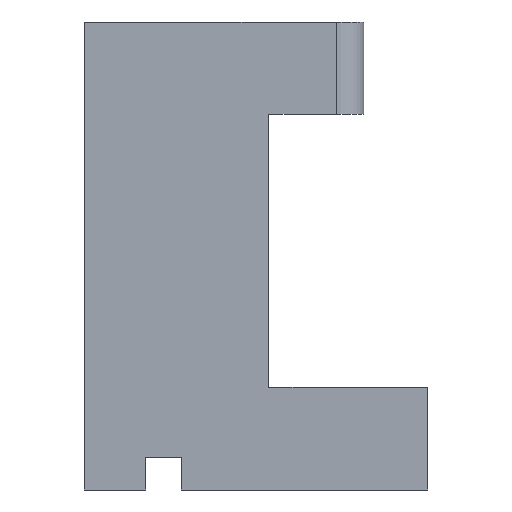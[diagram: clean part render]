
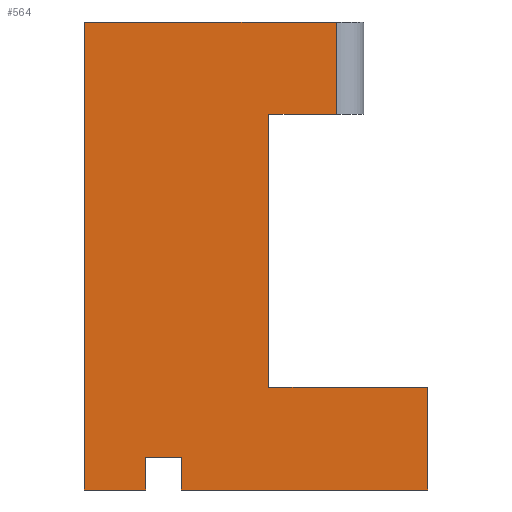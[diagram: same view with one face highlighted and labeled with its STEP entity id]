
A CAD part, front view. The second image highlights one B-rep face of the part: STEP entity #564.
In plain terms, the highlighted planar face has unit normal (0, -1, 0).
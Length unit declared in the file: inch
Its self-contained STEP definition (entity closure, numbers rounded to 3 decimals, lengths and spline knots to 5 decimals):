
#36=FACE_OUTER_BOUND('',#66,.T.);
#66=EDGE_LOOP('',(#399,#400,#401,#402,#403,#404,#405,#406,#407,#408,#409,
#410));
#125=LINE('',#836,#185);
#139=LINE('',#864,#199);
#140=LINE('',#866,#200);
#141=LINE('',#868,#201);
#142=LINE('',#870,#202);
#143=LINE('',#872,#203);
#144=LINE('',#874,#204);
#145=LINE('',#876,#205);
#146=LINE('',#878,#206);
#147=LINE('',#880,#207);
#148=LINE('',#882,#208);
#149=LINE('',#883,#209);
#185=VECTOR('',#669,0.3937);
#199=VECTOR('',#687,0.3937);
#200=VECTOR('',#688,0.3937);
#201=VECTOR('',#689,0.3937);
#202=VECTOR('',#690,0.3937);
#203=VECTOR('',#691,0.3937);
#204=VECTOR('',#692,0.3937);
#205=VECTOR('',#693,0.3937);
#206=VECTOR('',#694,0.3937);
#207=VECTOR('',#695,0.3937);
#208=VECTOR('',#696,0.3937);
#209=VECTOR('',#697,0.3937);
#246=VERTEX_POINT('',#832);
#248=VERTEX_POINT('',#835);
#260=VERTEX_POINT('',#863);
#261=VERTEX_POINT('',#865);
#262=VERTEX_POINT('',#867);
#263=VERTEX_POINT('',#869);
#264=VERTEX_POINT('',#871);
#265=VERTEX_POINT('',#873);
#266=VERTEX_POINT('',#875);
#267=VERTEX_POINT('',#877);
#268=VERTEX_POINT('',#879);
#269=VERTEX_POINT('',#881);
#302=EDGE_CURVE('',#248,#246,#125,.T.);
#316=EDGE_CURVE('',#260,#248,#139,.T.);
#317=EDGE_CURVE('',#261,#246,#140,.T.);
#318=EDGE_CURVE('',#261,#262,#141,.T.);
#319=EDGE_CURVE('',#262,#263,#142,.T.);
#320=EDGE_CURVE('',#263,#264,#143,.T.);
#321=EDGE_CURVE('',#265,#264,#144,.T.);
#322=EDGE_CURVE('',#265,#266,#145,.T.);
#323=EDGE_CURVE('',#266,#267,#146,.T.);
#324=EDGE_CURVE('',#267,#268,#147,.T.);
#325=EDGE_CURVE('',#269,#268,#148,.T.);
#326=EDGE_CURVE('',#260,#269,#149,.T.);
#399=ORIENTED_EDGE('',*,*,#316,.T.);
#400=ORIENTED_EDGE('',*,*,#302,.T.);
#401=ORIENTED_EDGE('',*,*,#317,.F.);
#402=ORIENTED_EDGE('',*,*,#318,.T.);
#403=ORIENTED_EDGE('',*,*,#319,.T.);
#404=ORIENTED_EDGE('',*,*,#320,.T.);
#405=ORIENTED_EDGE('',*,*,#321,.F.);
#406=ORIENTED_EDGE('',*,*,#322,.T.);
#407=ORIENTED_EDGE('',*,*,#323,.T.);
#408=ORIENTED_EDGE('',*,*,#324,.T.);
#409=ORIENTED_EDGE('',*,*,#325,.F.);
#410=ORIENTED_EDGE('',*,*,#326,.F.);
#545=PLANE('',#609);
#564=ADVANCED_FACE('',(#36),#545,.T.);
#609=AXIS2_PLACEMENT_3D('',#862,#685,#686);
#669=DIRECTION('',(0.,0.,1.));
#685=DIRECTION('center_axis',(0.,-1.,0.));
#686=DIRECTION('ref_axis',(0.,0.,-1.));
#687=DIRECTION('',(-1.,0.,0.));
#688=DIRECTION('',(-1.,0.,0.));
#689=DIRECTION('',(0.,0.,1.));
#690=DIRECTION('',(-1.,0.,0.));
#691=DIRECTION('',(0.,0.,-1.));
#692=DIRECTION('',(-1.,0.,0.));
#693=DIRECTION('',(0.,0.,1.));
#694=DIRECTION('',(1.,0.,0.));
#695=DIRECTION('',(0.,0.,-1.));
#696=DIRECTION('',(-1.,0.,0.));
#697=DIRECTION('',(0.,0.,-1.));
#832=CARTESIAN_POINT('',(-9.86369,-2.02165,3.12));
#835=CARTESIAN_POINT('',(-9.86369,-2.02165,1.27));
#836=CARTESIAN_POINT('',(-9.86369,-2.02165,1.70441));
#862=CARTESIAN_POINT('Origin',(-10.08567,-2.02165,2.08381));
#863=CARTESIAN_POINT('',(-8.78869,-2.02165,1.27));
#864=CARTESIAN_POINT('',(-9.93718,-2.02165,1.27));
#865=CARTESIAN_POINT('',(-9.40669,-2.02165,3.12));
#866=CARTESIAN_POINT('',(-9.15669,-2.02165,3.12));
#867=CARTESIAN_POINT('',(-9.40669,-2.02165,3.745));
#868=CARTESIAN_POINT('',(-9.40669,-2.02165,3.8));
#869=CARTESIAN_POINT('',(-11.11339,-2.02165,3.745));
#870=CARTESIAN_POINT('',(-9.62118,-2.02165,3.745));
#871=CARTESIAN_POINT('',(-11.11339,-2.02165,0.575));
#872=CARTESIAN_POINT('',(-11.11339,-2.02165,2.94191));
#873=CARTESIAN_POINT('',(-10.69803,-2.02165,0.575));
#874=CARTESIAN_POINT('',(-10.60868,-2.02165,0.575));
#875=CARTESIAN_POINT('',(-10.69803,-2.02165,0.79626));
#876=CARTESIAN_POINT('',(-10.69803,-2.02165,1.29004));
#877=CARTESIAN_POINT('',(-10.45669,-2.02165,0.79626));
#878=CARTESIAN_POINT('',(-10.33152,-2.02165,0.79626));
#879=CARTESIAN_POINT('',(-10.45669,-2.02165,0.575));
#880=CARTESIAN_POINT('',(-10.45669,-2.02165,1.29004));
#881=CARTESIAN_POINT('',(-8.78869,-2.02165,0.575));
#882=CARTESIAN_POINT('',(-10.27118,-2.02165,0.575));
#883=CARTESIAN_POINT('',(-8.78869,-2.02165,1.325));
